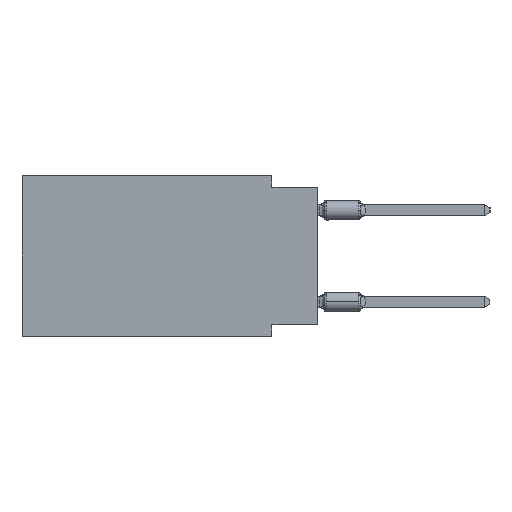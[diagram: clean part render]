
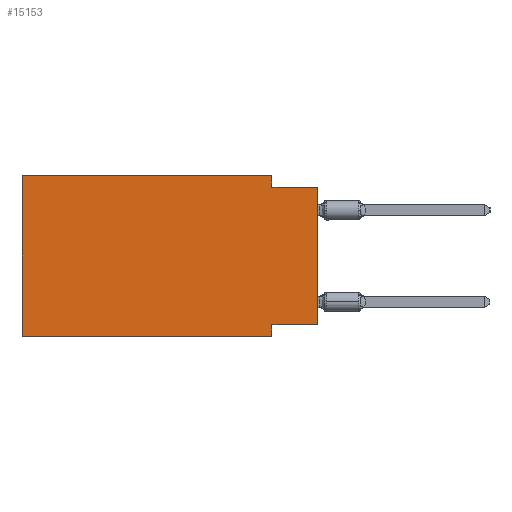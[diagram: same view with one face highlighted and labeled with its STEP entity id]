
A CAD part, left-side view. The second image highlights one B-rep face of the part: STEP entity #15153.
In plain terms, the highlighted planar face has unit normal (-1, 0, 0).
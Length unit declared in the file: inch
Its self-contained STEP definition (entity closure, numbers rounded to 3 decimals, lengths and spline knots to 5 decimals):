
#2658 = VERTEX_POINT ( 'NONE', #20284 ) ;
#4726 = EDGE_LOOP ( 'NONE', ( #14951, #19461, #32893, #52178, #17465, #27307, #54515, #16725 ) ) ;
#5783 = VECTOR ( 'NONE', #50854, 39.37008 ) ;
#5902 = VERTEX_POINT ( 'NONE', #18705 ) ;
#6550 = CARTESIAN_POINT ( 'NONE',  ( 0., 0., -0.025 ) ) ;
#7340 = CARTESIAN_POINT ( 'NONE',  ( 0., 0.1, -0.35 ) ) ;
#7501 = DIRECTION ( 'NONE',  ( 0., 0., 1. ) ) ;
#9099 = VERTEX_POINT ( 'NONE', #15915 ) ;
#10848 = DIRECTION ( 'NONE',  ( 0., -1., 0. ) ) ;
#11016 = VECTOR ( 'NONE', #41978, 39.37008 ) ;
#12429 = LINE ( 'NONE', #33501, #48096 ) ;
#13602 = CARTESIAN_POINT ( 'NONE',  ( 0., 0.1, -0.35 ) ) ;
#14951 = ORIENTED_EDGE ( 'NONE', *, *, #25745, .T. ) ;
#15153 = ADVANCED_FACE ( 'NONE', ( #17535 ), #17270, .F. ) ;
#15915 = CARTESIAN_POINT ( 'NONE',  ( 0., 0.645, -0.35 ) ) ;
#16698 = CARTESIAN_POINT ( 'NONE',  ( 0., 0., -0.025 ) ) ;
#16725 = ORIENTED_EDGE ( 'NONE', *, *, #18385, .F. ) ;
#16838 = LINE ( 'NONE', #25943, #5783 ) ;
#17270 = PLANE ( 'NONE',  #40840 ) ;
#17465 = ORIENTED_EDGE ( 'NONE', *, *, #19930, .F. ) ;
#17535 = FACE_OUTER_BOUND ( 'NONE', #4726, .T. ) ;
#18385 = EDGE_CURVE ( 'NONE', #5902, #35767, #16838, .T. ) ;
#18593 = EDGE_CURVE ( 'NONE', #36140, #26755, #27585, .T. ) ;
#18705 = CARTESIAN_POINT ( 'NONE',  ( 0., 0., -0.325 ) ) ;
#19461 = ORIENTED_EDGE ( 'NONE', *, *, #18593, .F. ) ;
#19930 = EDGE_CURVE ( 'NONE', #9099, #54123, #26372, .T. ) ;
#20284 = CARTESIAN_POINT ( 'NONE',  ( 0., 0.1, 0. ) ) ;
#21049 = VECTOR ( 'NONE', #10848, 39.37008 ) ;
#21955 = CARTESIAN_POINT ( 'NONE',  ( 0., 0.645, 0. ) ) ;
#23560 = EDGE_CURVE ( 'NONE', #54123, #2658, #32717, .T. ) ;
#25745 = EDGE_CURVE ( 'NONE', #5902, #26755, #32703, .T. ) ;
#25943 = CARTESIAN_POINT ( 'NONE',  ( 0., 0., -0.325 ) ) ;
#26372 = LINE ( 'NONE', #21955, #11016 ) ;
#26755 = VERTEX_POINT ( 'NONE', #16698 ) ;
#27307 = ORIENTED_EDGE ( 'NONE', *, *, #44163, .T. ) ;
#27585 = LINE ( 'NONE', #6550, #31476 ) ;
#27776 = CARTESIAN_POINT ( 'NONE',  ( 0., 0.1, -0.025 ) ) ;
#28659 = CARTESIAN_POINT ( 'NONE',  ( 0., 0.1, -0.325 ) ) ;
#31476 = VECTOR ( 'NONE', #45019, 39.37008 ) ;
#32703 = LINE ( 'NONE', #49552, #48650 ) ;
#32717 = LINE ( 'NONE', #49313, #21049 ) ;
#32893 = ORIENTED_EDGE ( 'NONE', *, *, #53063, .F. ) ;
#33501 = CARTESIAN_POINT ( 'NONE',  ( 0., 0.645, -0.35 ) ) ;
#33599 = DIRECTION ( 'NONE',  ( 0., 0., -1. ) ) ;
#35767 = VERTEX_POINT ( 'NONE', #28659 ) ;
#36140 = VERTEX_POINT ( 'NONE', #27776 ) ;
#37393 = VERTEX_POINT ( 'NONE', #13602 ) ;
#38592 = DIRECTION ( 'NONE',  ( 1., 0., 0. ) ) ;
#39588 = VECTOR ( 'NONE', #40581, 39.37008 ) ;
#40581 = DIRECTION ( 'NONE',  ( 0., 0., -1. ) ) ;
#40840 = AXIS2_PLACEMENT_3D ( 'NONE', #46857, #38592, #33599 ) ;
#41978 = DIRECTION ( 'NONE',  ( 0., 0., 1. ) ) ;
#43685 = DIRECTION ( 'NONE',  ( 0., 0., -1. ) ) ;
#44163 = EDGE_CURVE ( 'NONE', #9099, #37393, #12429, .T. ) ;
#45019 = DIRECTION ( 'NONE',  ( 0., -1., 0. ) ) ;
#45255 = LINE ( 'NONE', #7340, #39588 ) ;
#46605 = CARTESIAN_POINT ( 'NONE',  ( 0., 0.645, 0. ) ) ;
#46789 = EDGE_CURVE ( 'NONE', #35767, #37393, #45255, .T. ) ;
#46857 = CARTESIAN_POINT ( 'NONE',  ( 0., 0.645, 0. ) ) ;
#46878 = VECTOR ( 'NONE', #43685, 39.37008 ) ;
#48096 = VECTOR ( 'NONE', #54220, 39.37008 ) ;
#48381 = LINE ( 'NONE', #48645, #46878 ) ;
#48645 = CARTESIAN_POINT ( 'NONE',  ( 0., 0.1, 0. ) ) ;
#48650 = VECTOR ( 'NONE', #7501, 39.37008 ) ;
#49313 = CARTESIAN_POINT ( 'NONE',  ( 0., 0.645, 0. ) ) ;
#49552 = CARTESIAN_POINT ( 'NONE',  ( 0., 0., 0. ) ) ;
#50854 = DIRECTION ( 'NONE',  ( 0., 1., 0. ) ) ;
#52178 = ORIENTED_EDGE ( 'NONE', *, *, #23560, .F. ) ;
#53063 = EDGE_CURVE ( 'NONE', #2658, #36140, #48381, .T. ) ;
#54123 = VERTEX_POINT ( 'NONE', #46605 ) ;
#54220 = DIRECTION ( 'NONE',  ( 0., -1., 0. ) ) ;
#54515 = ORIENTED_EDGE ( 'NONE', *, *, #46789, .F. ) ;
